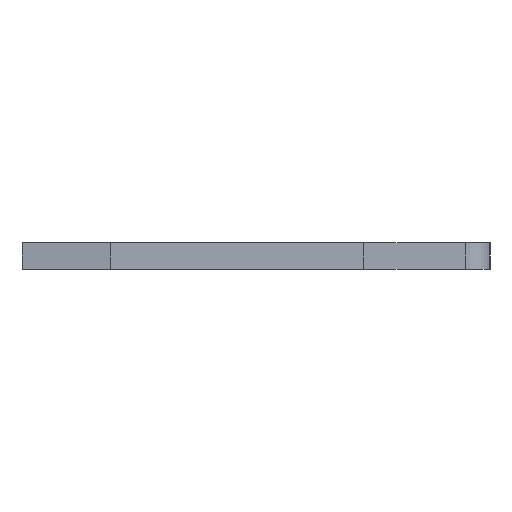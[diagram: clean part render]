
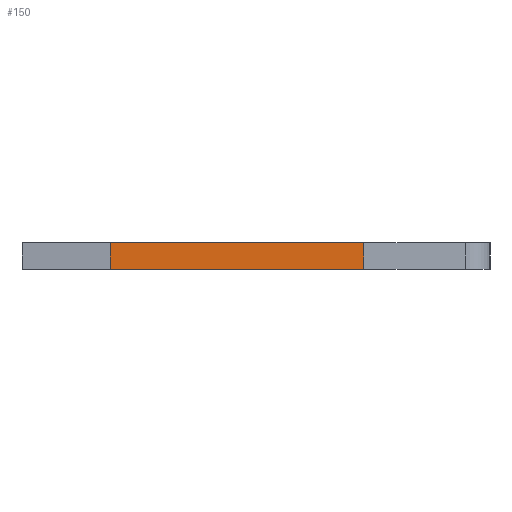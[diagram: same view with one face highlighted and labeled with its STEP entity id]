
A CAD part, left-side view. The second image highlights one B-rep face of the part: STEP entity #150.
In plain terms, the highlighted face is planar.
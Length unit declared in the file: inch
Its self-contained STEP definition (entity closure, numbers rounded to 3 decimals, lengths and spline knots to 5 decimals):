
#13 = LINE ( 'NONE', #989, #885 ) ;
#120 = ORIENTED_EDGE ( 'NONE', *, *, #1346, .F. ) ;
#142 = VERTEX_POINT ( 'NONE', #158 ) ;
#150 = ADVANCED_FACE ( 'NONE', ( #841 ), #1087, .F. ) ;
#158 = CARTESIAN_POINT ( 'NONE',  ( -0.013, 0.146, -0.0575 ) ) ;
#188 = VERTEX_POINT ( 'NONE', #1406 ) ;
#199 = DIRECTION ( 'NONE',  ( -1., 0., 0. ) ) ;
#214 = VERTEX_POINT ( 'NONE', #1723 ) ;
#277 = EDGE_CURVE ( 'NONE', #188, #142, #286, .T. ) ;
#286 = LINE ( 'NONE', #489, #1141 ) ;
#328 = DIRECTION ( 'NONE',  ( 0., 1., 0. ) ) ;
#336 = DIRECTION ( 'NONE',  ( 1., 0., 0. ) ) ;
#404 = ORIENTED_EDGE ( 'NONE', *, *, #277, .T. ) ;
#489 = CARTESIAN_POINT ( 'NONE',  ( -0.013, 0.146, -0.0575 ) ) ;
#558 = DIRECTION ( 'NONE',  ( -1., 0., 0. ) ) ;
#671 = EDGE_LOOP ( 'NONE', ( #404, #120, #1513, #889 ) ) ;
#764 = LINE ( 'NONE', #1281, #1535 ) ;
#827 = EDGE_CURVE ( 'NONE', #1953, #214, #13, .T. ) ;
#841 = FACE_OUTER_BOUND ( 'NONE', #671, .T. ) ;
#885 = VECTOR ( 'NONE', #995, 39.37008 ) ;
#889 = ORIENTED_EDGE ( 'NONE', *, *, #1909, .T. ) ;
#989 = CARTESIAN_POINT ( 'NONE',  ( 0.013, 0.146, -0.0575 ) ) ;
#995 = DIRECTION ( 'NONE',  ( 0., 1., 0. ) ) ;
#1029 = CARTESIAN_POINT ( 'NONE',  ( 0.013, 0.146, -0.0575 ) ) ;
#1087 = PLANE ( 'NONE',  #1231 ) ;
#1093 = CARTESIAN_POINT ( 'NONE',  ( 0.013, 0.146, -0.0575 ) ) ;
#1111 = CARTESIAN_POINT ( 'NONE',  ( 0.013, -0.099, -0.0575 ) ) ;
#1141 = VECTOR ( 'NONE', #328, 39.37008 ) ;
#1211 = VECTOR ( 'NONE', #558, 39.37008 ) ;
#1231 = AXIS2_PLACEMENT_3D ( 'NONE', #1093, #1378, #336 ) ;
#1281 = CARTESIAN_POINT ( 'NONE',  ( 0.013, -0.099, -0.0575 ) ) ;
#1346 = EDGE_CURVE ( 'NONE', #214, #142, #1778, .T. ) ;
#1378 = DIRECTION ( 'NONE',  ( 0., 0., 1. ) ) ;
#1406 = CARTESIAN_POINT ( 'NONE',  ( -0.013, -0.099, -0.0575 ) ) ;
#1513 = ORIENTED_EDGE ( 'NONE', *, *, #827, .F. ) ;
#1535 = VECTOR ( 'NONE', #199, 39.37008 ) ;
#1723 = CARTESIAN_POINT ( 'NONE',  ( 0.013, 0.146, -0.0575 ) ) ;
#1778 = LINE ( 'NONE', #1029, #1211 ) ;
#1909 = EDGE_CURVE ( 'NONE', #1953, #188, #764, .T. ) ;
#1953 = VERTEX_POINT ( 'NONE', #1111 ) ;
